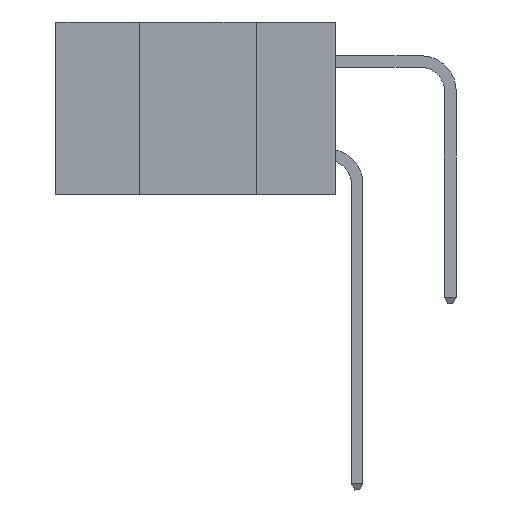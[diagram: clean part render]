
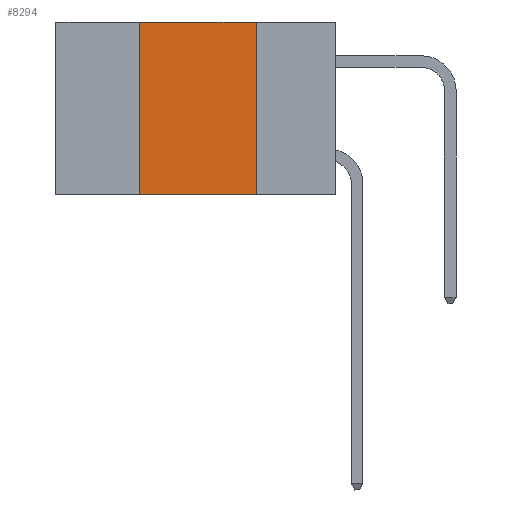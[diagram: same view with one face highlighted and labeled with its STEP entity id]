
A CAD part, left-side view. The second image highlights one B-rep face of the part: STEP entity #8294.
In plain terms, the highlighted planar face has unit normal (-1, 0, 0).
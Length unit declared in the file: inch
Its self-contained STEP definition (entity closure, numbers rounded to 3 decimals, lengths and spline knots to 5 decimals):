
#381 = CARTESIAN_POINT ( 'NONE',  ( 0., 0.42, 0. ) ) ;
#449 = CARTESIAN_POINT ( 'NONE',  ( 0., 0.17, 0. ) ) ;
#667 = CARTESIAN_POINT ( 'NONE',  ( 0., 0.6, -0.37 ) ) ;
#692 = FACE_OUTER_BOUND ( 'NONE', #5287, .T. ) ;
#830 = LINE ( 'NONE', #667, #20191 ) ;
#964 = VECTOR ( 'NONE', #11743, 39.37008 ) ;
#1342 = CARTESIAN_POINT ( 'NONE',  ( 0., 0.42, 0. ) ) ;
#3325 = LINE ( 'NONE', #449, #964 ) ;
#3584 = VERTEX_POINT ( 'NONE', #15130 ) ;
#4971 = ORIENTED_EDGE ( 'NONE', *, *, #17802, .F. ) ;
#5287 = EDGE_LOOP ( 'NONE', ( #4971, #14912, #21515, #18187 ) ) ;
#6552 = DIRECTION ( 'NONE',  ( 0., -1., 0. ) ) ;
#7064 = DIRECTION ( 'NONE',  ( 1., 0., 0. ) ) ;
#8294 = ADVANCED_FACE ( 'NONE', ( #692 ), #21915, .F. ) ;
#10038 = CARTESIAN_POINT ( 'NONE',  ( 0., 0.42, -0.37 ) ) ;
#10333 = DIRECTION ( 'NONE',  ( 0., -1., 0. ) ) ;
#10685 = DIRECTION ( 'NONE',  ( 0., 0., -1. ) ) ;
#11004 = AXIS2_PLACEMENT_3D ( 'NONE', #16477, #7064, #10685 ) ;
#11438 = CARTESIAN_POINT ( 'NONE',  ( 0., 0.17, -0.37 ) ) ;
#11571 = VECTOR ( 'NONE', #14457, 39.37008 ) ;
#11743 = DIRECTION ( 'NONE',  ( 0., 0., -1. ) ) ;
#14444 = VERTEX_POINT ( 'NONE', #381 ) ;
#14457 = DIRECTION ( 'NONE',  ( 0., 0., 1. ) ) ;
#14912 = ORIENTED_EDGE ( 'NONE', *, *, #21933, .F. ) ;
#15130 = CARTESIAN_POINT ( 'NONE',  ( 0., 0.17, 0. ) ) ;
#15949 = EDGE_CURVE ( 'NONE', #23756, #23093, #830, .T. ) ;
#16353 = VECTOR ( 'NONE', #10333, 39.37008 ) ;
#16477 = CARTESIAN_POINT ( 'NONE',  ( 0., 0.6, 0. ) ) ;
#16842 = EDGE_CURVE ( 'NONE', #23756, #14444, #19471, .T. ) ;
#17802 = EDGE_CURVE ( 'NONE', #3584, #23093, #3325, .T. ) ;
#18187 = ORIENTED_EDGE ( 'NONE', *, *, #15949, .T. ) ;
#19471 = LINE ( 'NONE', #1342, #11571 ) ;
#20191 = VECTOR ( 'NONE', #6552, 39.37008 ) ;
#21515 = ORIENTED_EDGE ( 'NONE', *, *, #16842, .F. ) ;
#21915 = PLANE ( 'NONE',  #11004 ) ;
#21933 = EDGE_CURVE ( 'NONE', #14444, #3584, #24015, .T. ) ;
#22552 = CARTESIAN_POINT ( 'NONE',  ( 0., 0.6, 0. ) ) ;
#23093 = VERTEX_POINT ( 'NONE', #11438 ) ;
#23756 = VERTEX_POINT ( 'NONE', #10038 ) ;
#24015 = LINE ( 'NONE', #22552, #16353 ) ;
